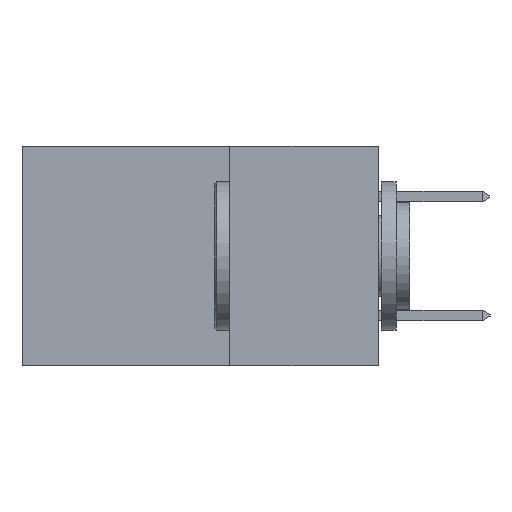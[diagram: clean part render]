
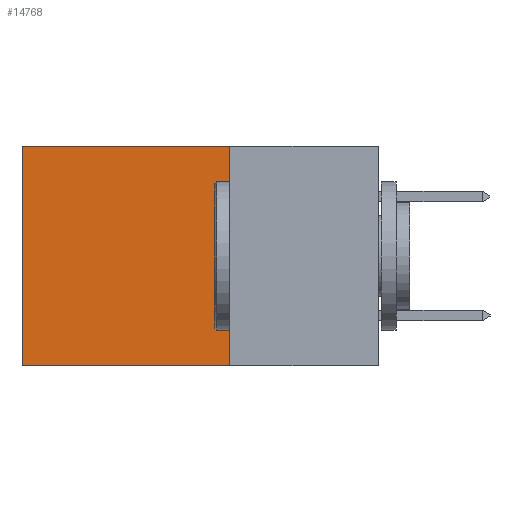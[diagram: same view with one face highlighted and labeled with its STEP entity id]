
A CAD part, left-side view. The second image highlights one B-rep face of the part: STEP entity #14768.
In plain terms, the highlighted planar face has unit normal (-1, 0, 0).
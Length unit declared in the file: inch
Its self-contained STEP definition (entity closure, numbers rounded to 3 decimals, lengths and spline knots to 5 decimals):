
#311 = EDGE_CURVE ( 'NONE', #2087, #10345, #2194, .T. ) ;
#477 = VERTEX_POINT ( 'NONE', #13645 ) ;
#1279 = ORIENTED_EDGE ( 'NONE', *, *, #311, .F. ) ;
#1710 = CARTESIAN_POINT ( 'NONE',  ( 0.2615, 0.25, -0.37 ) ) ;
#1805 = FACE_OUTER_BOUND ( 'NONE', #2338, .T. ) ;
#2087 = VERTEX_POINT ( 'NONE', #9609 ) ;
#2194 = LINE ( 'NONE', #8160, #13800 ) ;
#2338 = EDGE_LOOP ( 'NONE', ( #5196, #10031, #1279, #3728 ) ) ;
#2791 = CARTESIAN_POINT ( 'NONE',  ( 0.2615, 0.6, -0.37 ) ) ;
#2849 = DIRECTION ( 'NONE',  ( 0., 0., -1. ) ) ;
#3632 = VECTOR ( 'NONE', #7946, 39.37008 ) ;
#3728 = ORIENTED_EDGE ( 'NONE', *, *, #5152, .T. ) ;
#4837 = VECTOR ( 'NONE', #11391, 39.37008 ) ;
#4907 = LINE ( 'NONE', #2791, #10435 ) ;
#5152 = EDGE_CURVE ( 'NONE', #2087, #9688, #6854, .T. ) ;
#5196 = ORIENTED_EDGE ( 'NONE', *, *, #7015, .T. ) ;
#6854 = LINE ( 'NONE', #8050, #3632 ) ;
#6970 = AXIS2_PLACEMENT_3D ( 'NONE', #7362, #14742, #8454 ) ;
#7015 = EDGE_CURVE ( 'NONE', #9688, #477, #4907, .T. ) ;
#7362 = CARTESIAN_POINT ( 'NONE',  ( 0.2615, 0.25, -0.37 ) ) ;
#7946 = DIRECTION ( 'NONE',  ( 0., 1., 0. ) ) ;
#8050 = CARTESIAN_POINT ( 'NONE',  ( 0.2615, 0.25, 0. ) ) ;
#8160 = CARTESIAN_POINT ( 'NONE',  ( 0.2615, 0.25, -0.37 ) ) ;
#8454 = DIRECTION ( 'NONE',  ( 0., 0., -1. ) ) ;
#9325 = CARTESIAN_POINT ( 'NONE',  ( 0.2615, 0.25, -0.37 ) ) ;
#9609 = CARTESIAN_POINT ( 'NONE',  ( 0.2615, 0.25, 0. ) ) ;
#9688 = VERTEX_POINT ( 'NONE', #11890 ) ;
#9926 = EDGE_CURVE ( 'NONE', #10345, #477, #14950, .T. ) ;
#10031 = ORIENTED_EDGE ( 'NONE', *, *, #9926, .F. ) ;
#10345 = VERTEX_POINT ( 'NONE', #1710 ) ;
#10435 = VECTOR ( 'NONE', #2849, 39.37008 ) ;
#10814 = DIRECTION ( 'NONE',  ( 0., 0., -1. ) ) ;
#11391 = DIRECTION ( 'NONE',  ( 0., 1., 0. ) ) ;
#11890 = CARTESIAN_POINT ( 'NONE',  ( 0.2615, 0.6, 0. ) ) ;
#12653 = PLANE ( 'NONE',  #6970 ) ;
#13645 = CARTESIAN_POINT ( 'NONE',  ( 0.2615, 0.6, -0.37 ) ) ;
#13800 = VECTOR ( 'NONE', #10814, 39.37008 ) ;
#14742 = DIRECTION ( 'NONE',  ( 1., 0., 0. ) ) ;
#14768 = ADVANCED_FACE ( 'NONE', ( #1805 ), #12653, .F. ) ;
#14950 = LINE ( 'NONE', #9325, #4837 ) ;
